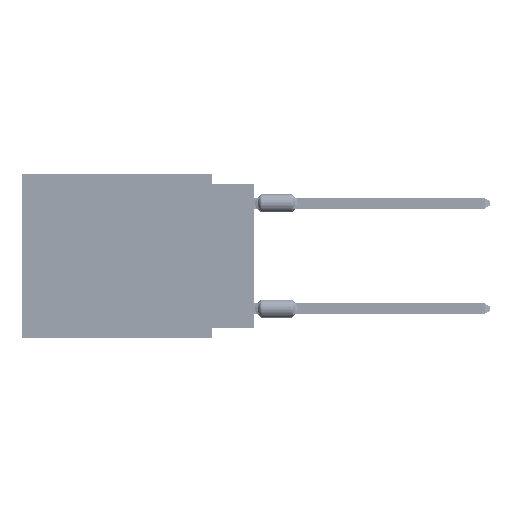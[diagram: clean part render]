
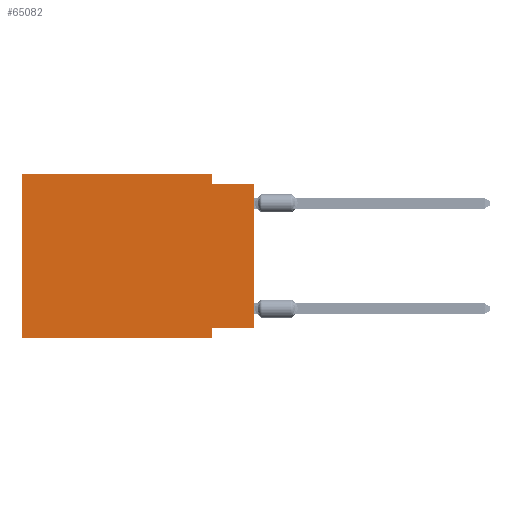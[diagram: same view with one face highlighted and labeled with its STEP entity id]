
A CAD part, left-side view. The second image highlights one B-rep face of the part: STEP entity #65082.
In plain terms, the highlighted planar face has unit normal (-1, 0, 0).
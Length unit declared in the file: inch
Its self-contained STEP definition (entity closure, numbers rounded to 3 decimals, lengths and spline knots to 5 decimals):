
#260 = VERTEX_POINT ( 'NONE', #4381 ) ;
#1034 = DIRECTION ( 'NONE',  ( 0., 1., 0. ) ) ;
#1739 = CARTESIAN_POINT ( 'NONE',  ( 0., 0.1, -0.39 ) ) ;
#2024 = VECTOR ( 'NONE', #19498, 39.37008 ) ;
#2327 = CARTESIAN_POINT ( 'NONE',  ( 0., 0.55, -0.39 ) ) ;
#3611 = CARTESIAN_POINT ( 'NONE',  ( 0., 0.55, -0.39 ) ) ;
#4381 = CARTESIAN_POINT ( 'NONE',  ( 0., 0., -0.025 ) ) ;
#4641 = VECTOR ( 'NONE', #20297, 39.37008 ) ;
#5174 = VERTEX_POINT ( 'NONE', #57734 ) ;
#6044 = CARTESIAN_POINT ( 'NONE',  ( 0., 0.55, 0. ) ) ;
#7174 = ORIENTED_EDGE ( 'NONE', *, *, #28270, .F. ) ;
#8445 = ORIENTED_EDGE ( 'NONE', *, *, #62095, .T. ) ;
#9718 = CARTESIAN_POINT ( 'NONE',  ( 0., 0., 0. ) ) ;
#12871 = FACE_OUTER_BOUND ( 'NONE', #24426, .T. ) ;
#13654 = EDGE_CURVE ( 'NONE', #31312, #34822, #46073, .T. ) ;
#13859 = EDGE_CURVE ( 'NONE', #30304, #5174, #47148, .T. ) ;
#15402 = VECTOR ( 'NONE', #28190, 39.37008 ) ;
#17947 = PLANE ( 'NONE',  #31281 ) ;
#19498 = DIRECTION ( 'NONE',  ( 0., -1., 0. ) ) ;
#19567 = CARTESIAN_POINT ( 'NONE',  ( 0., 0.55, 0. ) ) ;
#20297 = DIRECTION ( 'NONE',  ( 0., -1., 0. ) ) ;
#20814 = DIRECTION ( 'NONE',  ( 0., -1., 0. ) ) ;
#20994 = LINE ( 'NONE', #9718, #39188 ) ;
#23414 = CARTESIAN_POINT ( 'NONE',  ( 0., 0.55, 0. ) ) ;
#24426 = EDGE_LOOP ( 'NONE', ( #8445, #7174, #36733, #59580, #26167, #26438, #29642, #39636 ) ) ;
#25023 = CARTESIAN_POINT ( 'NONE',  ( 0., 0.1, -0.365 ) ) ;
#26167 = ORIENTED_EDGE ( 'NONE', *, *, #70343, .F. ) ;
#26438 = ORIENTED_EDGE ( 'NONE', *, *, #35003, .T. ) ;
#27020 = CARTESIAN_POINT ( 'NONE',  ( 0., 0., -0.365 ) ) ;
#27701 = CARTESIAN_POINT ( 'NONE',  ( 0., 0.1, 0. ) ) ;
#28190 = DIRECTION ( 'NONE',  ( 0., 0., 1. ) ) ;
#28270 = EDGE_CURVE ( 'NONE', #49763, #260, #59401, .T. ) ;
#28991 = CARTESIAN_POINT ( 'NONE',  ( 0., 0., -0.365 ) ) ;
#29642 = ORIENTED_EDGE ( 'NONE', *, *, #61649, .F. ) ;
#30304 = VERTEX_POINT ( 'NONE', #19567 ) ;
#30557 = VERTEX_POINT ( 'NONE', #1739 ) ;
#31281 = AXIS2_PLACEMENT_3D ( 'NONE', #23414, #46663, #52123 ) ;
#31312 = VERTEX_POINT ( 'NONE', #27020 ) ;
#32647 = LINE ( 'NONE', #3611, #4641 ) ;
#34822 = VERTEX_POINT ( 'NONE', #25023 ) ;
#35003 = EDGE_CURVE ( 'NONE', #39823, #30557, #32647, .T. ) ;
#36733 = ORIENTED_EDGE ( 'NONE', *, *, #44364, .F. ) ;
#39188 = VECTOR ( 'NONE', #70085, 39.37008 ) ;
#39636 = ORIENTED_EDGE ( 'NONE', *, *, #13654, .F. ) ;
#39823 = VERTEX_POINT ( 'NONE', #2327 ) ;
#43698 = LINE ( 'NONE', #27701, #68035 ) ;
#43949 = VECTOR ( 'NONE', #20814, 39.37008 ) ;
#44364 = EDGE_CURVE ( 'NONE', #5174, #49763, #43698, .T. ) ;
#46073 = LINE ( 'NONE', #28991, #58949 ) ;
#46663 = DIRECTION ( 'NONE',  ( 1., 0., 0. ) ) ;
#47148 = LINE ( 'NONE', #52611, #2024 ) ;
#49546 = DIRECTION ( 'NONE',  ( 0., 0., -1. ) ) ;
#49763 = VERTEX_POINT ( 'NONE', #70830 ) ;
#50712 = DIRECTION ( 'NONE',  ( 0., 0., -1. ) ) ;
#51817 = LINE ( 'NONE', #6044, #15402 ) ;
#52123 = DIRECTION ( 'NONE',  ( 0., 0., -1. ) ) ;
#52611 = CARTESIAN_POINT ( 'NONE',  ( 0., 0.55, 0. ) ) ;
#55818 = CARTESIAN_POINT ( 'NONE',  ( 0., 0.1, -0.39 ) ) ;
#57734 = CARTESIAN_POINT ( 'NONE',  ( 0., 0.1, 0. ) ) ;
#58949 = VECTOR ( 'NONE', #1034, 39.37008 ) ;
#59401 = LINE ( 'NONE', #69558, #43949 ) ;
#59580 = ORIENTED_EDGE ( 'NONE', *, *, #13859, .F. ) ;
#61243 = VECTOR ( 'NONE', #50712, 39.37008 ) ;
#61649 = EDGE_CURVE ( 'NONE', #34822, #30557, #67053, .T. ) ;
#62095 = EDGE_CURVE ( 'NONE', #31312, #260, #20994, .T. ) ;
#65082 = ADVANCED_FACE ( 'NONE', ( #12871 ), #17947, .F. ) ;
#67053 = LINE ( 'NONE', #55818, #61243 ) ;
#68035 = VECTOR ( 'NONE', #49546, 39.37008 ) ;
#69558 = CARTESIAN_POINT ( 'NONE',  ( 0., 0., -0.025 ) ) ;
#70085 = DIRECTION ( 'NONE',  ( 0., 0., 1. ) ) ;
#70343 = EDGE_CURVE ( 'NONE', #39823, #30304, #51817, .T. ) ;
#70830 = CARTESIAN_POINT ( 'NONE',  ( 0., 0.1, -0.025 ) ) ;
